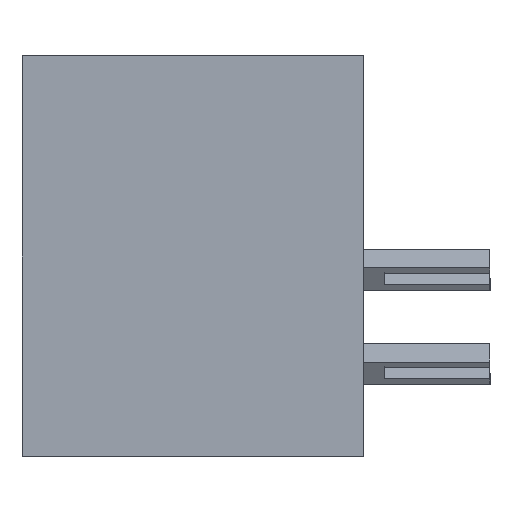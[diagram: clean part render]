
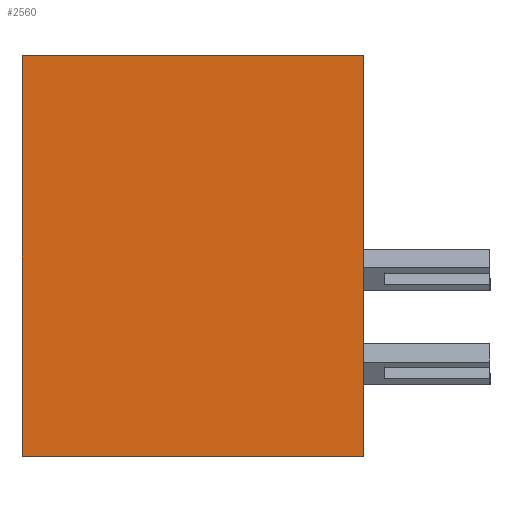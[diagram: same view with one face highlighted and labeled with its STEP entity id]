
A CAD part, left-side view. The second image highlights one B-rep face of the part: STEP entity #2560.
In plain terms, the highlighted planar face has unit normal (-1, 0, 0).
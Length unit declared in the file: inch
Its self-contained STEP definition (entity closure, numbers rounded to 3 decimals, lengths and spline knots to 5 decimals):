
#97 = VECTOR ( 'NONE', #2142, 39.37008 ) ;
#469 = LINE ( 'NONE', #11812, #10688 ) ;
#1045 = AXIS2_PLACEMENT_3D ( 'NONE', #5138, #12406, #6197 ) ;
#1469 = ORIENTED_EDGE ( 'NONE', *, *, #2305, .F. ) ;
#2142 = DIRECTION ( 'NONE',  ( 0., -1., 0. ) ) ;
#2305 = EDGE_CURVE ( 'NONE', #3128, #10852, #13346, .T. ) ;
#2560 = ADVANCED_FACE ( 'NONE', ( #9168 ), #14600, .F. ) ;
#2804 = VECTOR ( 'NONE', #3312, 39.37008 ) ;
#3128 = VERTEX_POINT ( 'NONE', #9589 ) ;
#3176 = VERTEX_POINT ( 'NONE', #4162 ) ;
#3312 = DIRECTION ( 'NONE',  ( 0., 0., 1. ) ) ;
#3357 = ORIENTED_EDGE ( 'NONE', *, *, #10660, .T. ) ;
#4162 = CARTESIAN_POINT ( 'NONE',  ( 0., 0., -0.531 ) ) ;
#5138 = CARTESIAN_POINT ( 'NONE',  ( 0., 0.453, 0. ) ) ;
#6197 = DIRECTION ( 'NONE',  ( 0., 0., -1. ) ) ;
#7253 = VECTOR ( 'NONE', #11759, 39.37008 ) ;
#8009 = CARTESIAN_POINT ( 'NONE',  ( 0., 0.453, 0. ) ) ;
#8331 = EDGE_CURVE ( 'NONE', #12007, #3128, #13394, .T. ) ;
#9054 = ORIENTED_EDGE ( 'NONE', *, *, #8331, .F. ) ;
#9168 = FACE_OUTER_BOUND ( 'NONE', #9772, .T. ) ;
#9589 = CARTESIAN_POINT ( 'NONE',  ( 0., 0.453, 0. ) ) ;
#9685 = CARTESIAN_POINT ( 'NONE',  ( 0., 0., 0. ) ) ;
#9772 = EDGE_LOOP ( 'NONE', ( #3357, #1469, #9054, #11311 ) ) ;
#10631 = EDGE_CURVE ( 'NONE', #12007, #3176, #13925, .T. ) ;
#10660 = EDGE_CURVE ( 'NONE', #3176, #10852, #469, .T. ) ;
#10688 = VECTOR ( 'NONE', #14171, 39.37008 ) ;
#10852 = VERTEX_POINT ( 'NONE', #9685 ) ;
#11311 = ORIENTED_EDGE ( 'NONE', *, *, #10631, .T. ) ;
#11759 = DIRECTION ( 'NONE',  ( 0., -1., 0. ) ) ;
#11812 = CARTESIAN_POINT ( 'NONE',  ( 0., 0., 0. ) ) ;
#12007 = VERTEX_POINT ( 'NONE', #14290 ) ;
#12406 = DIRECTION ( 'NONE',  ( 1., 0., 0. ) ) ;
#13089 = CARTESIAN_POINT ( 'NONE',  ( 0., 0.453, -0.531 ) ) ;
#13346 = LINE ( 'NONE', #8009, #97 ) ;
#13394 = LINE ( 'NONE', #14124, #2804 ) ;
#13925 = LINE ( 'NONE', #13089, #7253 ) ;
#14124 = CARTESIAN_POINT ( 'NONE',  ( 0., 0.453, 0. ) ) ;
#14171 = DIRECTION ( 'NONE',  ( 0., 0., 1. ) ) ;
#14290 = CARTESIAN_POINT ( 'NONE',  ( 0., 0.453, -0.531 ) ) ;
#14600 = PLANE ( 'NONE',  #1045 ) ;
